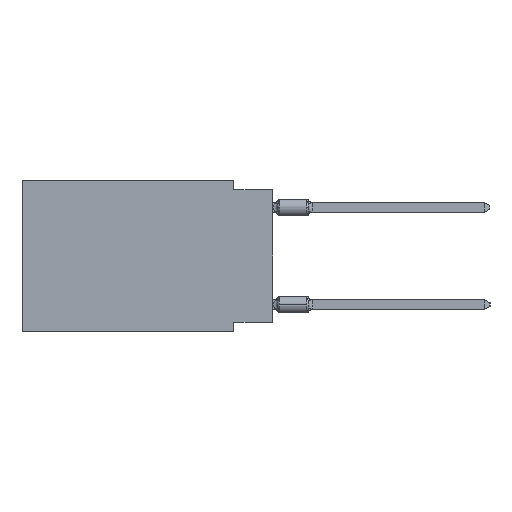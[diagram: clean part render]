
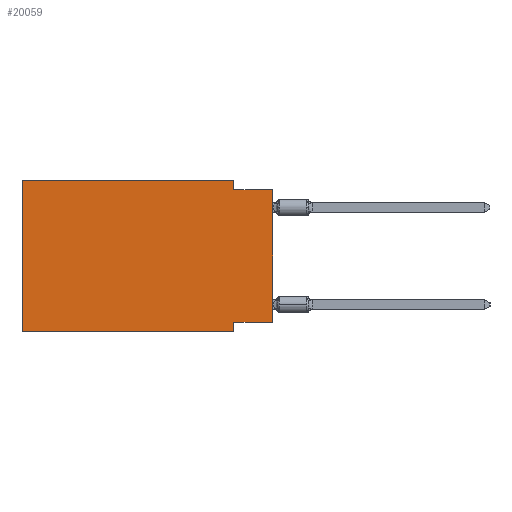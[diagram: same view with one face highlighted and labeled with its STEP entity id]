
A CAD part, left-side view. The second image highlights one B-rep face of the part: STEP entity #20059.
In plain terms, the highlighted planar face has unit normal (-1, 0, 0).
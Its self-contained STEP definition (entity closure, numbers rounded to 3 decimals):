
#1153 = PLANE ( 'NONE',  #2161 ) ;
#1481 = DIRECTION ( 'NONE',  ( 0., 0., -1. ) ) ;
#1625 = VECTOR ( 'NONE', #20694, 1000. ) ;
#1929 = EDGE_CURVE ( 'NONE', #29676, #21510, #17725, .T. ) ;
#2161 = AXIS2_PLACEMENT_3D ( 'NONE', #14391, #19885, #12334 ) ;
#2450 = CARTESIAN_POINT ( 'NONE',  ( 0., 16.383, -9.906 ) ) ;
#2468 = VECTOR ( 'NONE', #4994, 1000. ) ;
#3129 = CARTESIAN_POINT ( 'NONE',  ( 0., 0., 0. ) ) ;
#3822 = ORIENTED_EDGE ( 'NONE', *, *, #9374, .F. ) ;
#3828 = ORIENTED_EDGE ( 'NONE', *, *, #22130, .T. ) ;
#4212 = CARTESIAN_POINT ( 'NONE',  ( 0., 16.383, 0. ) ) ;
#4545 = ORIENTED_EDGE ( 'NONE', *, *, #8911, .T. ) ;
#4854 = LINE ( 'NONE', #2450, #22604 ) ;
#4994 = DIRECTION ( 'NONE',  ( 0., 1., 0. ) ) ;
#5522 = ORIENTED_EDGE ( 'NONE', *, *, #32745, .F. ) ;
#5941 = VECTOR ( 'NONE', #1481, 1000. ) ;
#5994 = VERTEX_POINT ( 'NONE', #31083 ) ;
#6181 = LINE ( 'NONE', #8428, #28166 ) ;
#8295 = DIRECTION ( 'NONE',  ( 0., 0., 1. ) ) ;
#8428 = CARTESIAN_POINT ( 'NONE',  ( 0., 16.383, 0. ) ) ;
#8473 = CARTESIAN_POINT ( 'NONE',  ( 0., 0., -9.271 ) ) ;
#8719 = CARTESIAN_POINT ( 'NONE',  ( 0., 2.54, -9.271 ) ) ;
#8911 = EDGE_CURVE ( 'NONE', #9980, #12858, #24087, .T. ) ;
#9374 = EDGE_CURVE ( 'NONE', #19757, #19542, #12325, .T. ) ;
#9980 = VERTEX_POINT ( 'NONE', #8473 ) ;
#10822 = VERTEX_POINT ( 'NONE', #31085 ) ;
#11909 = LINE ( 'NONE', #22397, #2468 ) ;
#12114 = LINE ( 'NONE', #4212, #1625 ) ;
#12325 = LINE ( 'NONE', #33127, #5941 ) ;
#12334 = DIRECTION ( 'NONE',  ( 0., 0., -1. ) ) ;
#12858 = VERTEX_POINT ( 'NONE', #13503 ) ;
#13178 = EDGE_CURVE ( 'NONE', #10822, #19757, #12114, .T. ) ;
#13503 = CARTESIAN_POINT ( 'NONE',  ( 0., 0., -0.635 ) ) ;
#14391 = CARTESIAN_POINT ( 'NONE',  ( 0., 16.383, 0. ) ) ;
#15943 = CARTESIAN_POINT ( 'NONE',  ( 0., 2.54, -9.906 ) ) ;
#16649 = DIRECTION ( 'NONE',  ( 0., 0., 1. ) ) ;
#17393 = DIRECTION ( 'NONE',  ( 0., -1., 0. ) ) ;
#17525 = ORIENTED_EDGE ( 'NONE', *, *, #29217, .F. ) ;
#17725 = LINE ( 'NONE', #23062, #30220 ) ;
#18362 = LINE ( 'NONE', #28710, #21864 ) ;
#19542 = VERTEX_POINT ( 'NONE', #24279 ) ;
#19757 = VERTEX_POINT ( 'NONE', #21270 ) ;
#19885 = DIRECTION ( 'NONE',  ( 1., 0., 0. ) ) ;
#20059 = ADVANCED_FACE ( 'NONE', ( #32956 ), #1153, .F. ) ;
#20694 = DIRECTION ( 'NONE',  ( 0., -1., 0. ) ) ;
#21270 = CARTESIAN_POINT ( 'NONE',  ( 0., 2.54, 0. ) ) ;
#21510 = VERTEX_POINT ( 'NONE', #15943 ) ;
#21864 = VECTOR ( 'NONE', #31094, 1000. ) ;
#22130 = EDGE_CURVE ( 'NONE', #5994, #21510, #4854, .T. ) ;
#22263 = EDGE_LOOP ( 'NONE', ( #4545, #22977, #3822, #31043, #17525, #3828, #32287, #5522 ) ) ;
#22397 = CARTESIAN_POINT ( 'NONE',  ( 0., 0., -9.271 ) ) ;
#22604 = VECTOR ( 'NONE', #17393, 1000. ) ;
#22977 = ORIENTED_EDGE ( 'NONE', *, *, #25346, .F. ) ;
#23062 = CARTESIAN_POINT ( 'NONE',  ( 0., 2.54, -9.906 ) ) ;
#23524 = VECTOR ( 'NONE', #8295, 1000. ) ;
#24087 = LINE ( 'NONE', #3129, #23524 ) ;
#24279 = CARTESIAN_POINT ( 'NONE',  ( 0., 2.54, -0.635 ) ) ;
#25346 = EDGE_CURVE ( 'NONE', #19542, #12858, #18362, .T. ) ;
#28053 = DIRECTION ( 'NONE',  ( 0., 0., -1. ) ) ;
#28166 = VECTOR ( 'NONE', #16649, 1000. ) ;
#28710 = CARTESIAN_POINT ( 'NONE',  ( 0., 0., -0.635 ) ) ;
#29217 = EDGE_CURVE ( 'NONE', #5994, #10822, #6181, .T. ) ;
#29676 = VERTEX_POINT ( 'NONE', #8719 ) ;
#30220 = VECTOR ( 'NONE', #28053, 1000. ) ;
#31043 = ORIENTED_EDGE ( 'NONE', *, *, #13178, .F. ) ;
#31083 = CARTESIAN_POINT ( 'NONE',  ( 0., 16.383, -9.906 ) ) ;
#31085 = CARTESIAN_POINT ( 'NONE',  ( 0., 16.383, 0. ) ) ;
#31094 = DIRECTION ( 'NONE',  ( 0., -1., 0. ) ) ;
#32287 = ORIENTED_EDGE ( 'NONE', *, *, #1929, .F. ) ;
#32745 = EDGE_CURVE ( 'NONE', #9980, #29676, #11909, .T. ) ;
#32956 = FACE_OUTER_BOUND ( 'NONE', #22263, .T. ) ;
#33127 = CARTESIAN_POINT ( 'NONE',  ( 0., 2.54, 0. ) ) ;
